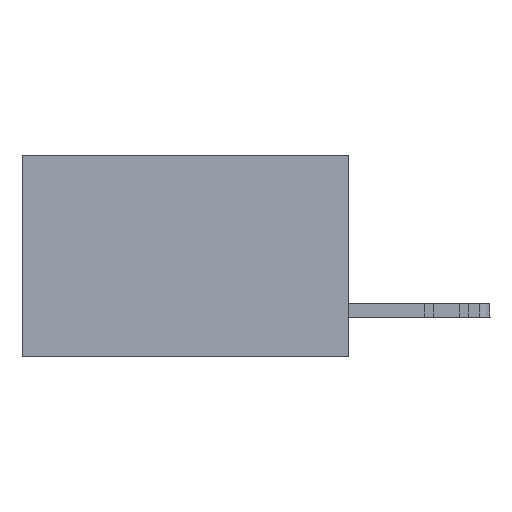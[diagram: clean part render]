
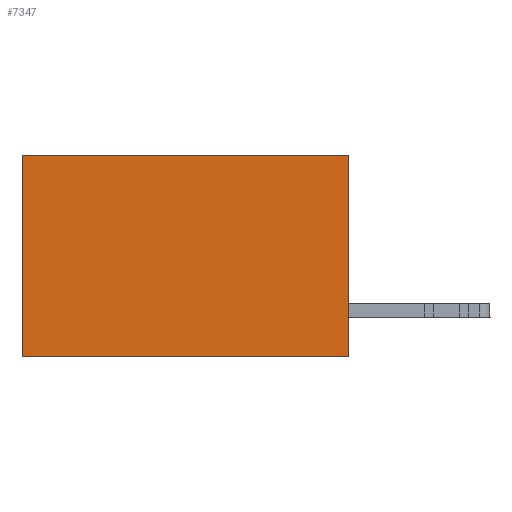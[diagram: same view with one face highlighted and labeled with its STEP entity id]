
A CAD part, left-side view. The second image highlights one B-rep face of the part: STEP entity #7347.
In plain terms, the highlighted planar face has unit normal (-1, 0, 0).
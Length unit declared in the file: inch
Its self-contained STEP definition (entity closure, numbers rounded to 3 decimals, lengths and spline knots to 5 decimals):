
#1248 = CARTESIAN_POINT ( 'NONE',  ( 0.298, 0., 0. ) ) ;
#1862 = VERTEX_POINT ( 'NONE', #10527 ) ;
#2810 = ORIENTED_EDGE ( 'NONE', *, *, #5681, .F. ) ;
#3375 = VERTEX_POINT ( 'NONE', #21085 ) ;
#4246 = DIRECTION ( 'NONE',  ( 0., 0., -1. ) ) ;
#4586 = CARTESIAN_POINT ( 'NONE',  ( 0.298, 0., -0.37 ) ) ;
#5681 = EDGE_CURVE ( 'NONE', #23865, #12308, #18773, .T. ) ;
#6401 = DIRECTION ( 'NONE',  ( 0., 0., -1. ) ) ;
#6453 = LINE ( 'NONE', #1248, #12296 ) ;
#6502 = DIRECTION ( 'NONE',  ( 1., 0., 0. ) ) ;
#7347 = ADVANCED_FACE ( 'NONE', ( #14132 ), #27734, .F. ) ;
#8609 = LINE ( 'NONE', #10069, #13332 ) ;
#10069 = CARTESIAN_POINT ( 'NONE',  ( 0.298, 0.6, 0. ) ) ;
#10527 = CARTESIAN_POINT ( 'NONE',  ( 0.298, 0., 0. ) ) ;
#11703 = ORIENTED_EDGE ( 'NONE', *, *, #14630, .T. ) ;
#12296 = VECTOR ( 'NONE', #22240, 39.37008 ) ;
#12308 = VERTEX_POINT ( 'NONE', #12756 ) ;
#12756 = CARTESIAN_POINT ( 'NONE',  ( 0.298, 0.6, -0.37 ) ) ;
#13332 = VECTOR ( 'NONE', #4246, 39.37008 ) ;
#13420 = CARTESIAN_POINT ( 'NONE',  ( 0.298, 0., 0. ) ) ;
#14132 = FACE_OUTER_BOUND ( 'NONE', #30189, .T. ) ;
#14282 = DIRECTION ( 'NONE',  ( 0., 0., -1. ) ) ;
#14630 = EDGE_CURVE ( 'NONE', #1862, #3375, #6453, .T. ) ;
#18083 = EDGE_CURVE ( 'NONE', #1862, #23865, #21530, .T. ) ;
#18773 = LINE ( 'NONE', #4586, #26139 ) ;
#19066 = CARTESIAN_POINT ( 'NONE',  ( 0.298, 0., 0. ) ) ;
#19316 = VECTOR ( 'NONE', #14282, 39.37008 ) ;
#21085 = CARTESIAN_POINT ( 'NONE',  ( 0.298, 0.6, 0. ) ) ;
#21530 = LINE ( 'NONE', #19066, #19316 ) ;
#22240 = DIRECTION ( 'NONE',  ( 0., 1., 0. ) ) ;
#22952 = DIRECTION ( 'NONE',  ( 0., 1., 0. ) ) ;
#23865 = VERTEX_POINT ( 'NONE', #30006 ) ;
#24999 = EDGE_CURVE ( 'NONE', #3375, #12308, #8609, .T. ) ;
#26076 = ORIENTED_EDGE ( 'NONE', *, *, #18083, .F. ) ;
#26139 = VECTOR ( 'NONE', #22952, 39.37008 ) ;
#26859 = ORIENTED_EDGE ( 'NONE', *, *, #24999, .T. ) ;
#27734 = PLANE ( 'NONE',  #28512 ) ;
#28512 = AXIS2_PLACEMENT_3D ( 'NONE', #13420, #6502, #6401 ) ;
#30006 = CARTESIAN_POINT ( 'NONE',  ( 0.298, 0., -0.37 ) ) ;
#30189 = EDGE_LOOP ( 'NONE', ( #26859, #2810, #26076, #11703 ) ) ;
